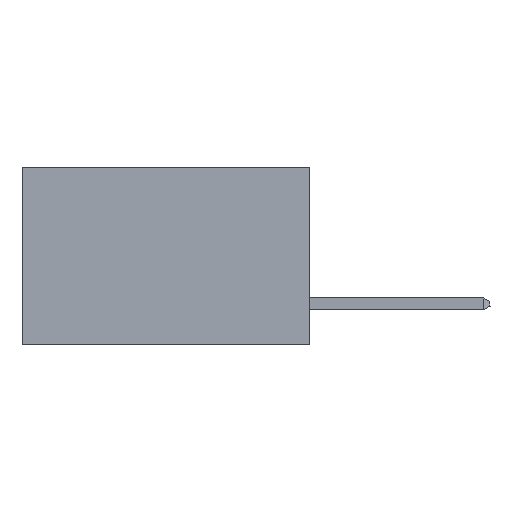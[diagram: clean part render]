
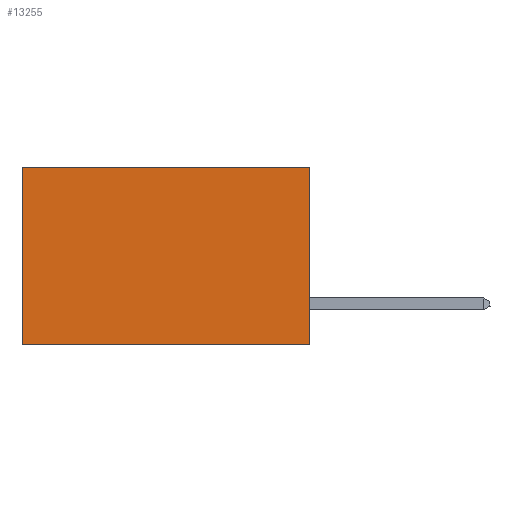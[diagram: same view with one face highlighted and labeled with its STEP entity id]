
A CAD part, left-side view. The second image highlights one B-rep face of the part: STEP entity #13255.
In plain terms, the highlighted planar face has unit normal (-1, 0, 0).
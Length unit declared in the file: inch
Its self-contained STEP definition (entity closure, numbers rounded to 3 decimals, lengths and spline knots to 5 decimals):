
#263 = LINE ( 'NONE', #4884, #8646 ) ;
#336 = VERTEX_POINT ( 'NONE', #20911 ) ;
#1980 = VECTOR ( 'NONE', #3413, 39.37008 ) ;
#2039 = VERTEX_POINT ( 'NONE', #3823 ) ;
#2098 = FACE_OUTER_BOUND ( 'NONE', #17016, .T. ) ;
#3413 = DIRECTION ( 'NONE',  ( 0., 1., 0. ) ) ;
#3480 = CARTESIAN_POINT ( 'NONE',  ( 0.2875, 0., -0.37 ) ) ;
#3809 = DIRECTION ( 'NONE',  ( 0., 0., -1. ) ) ;
#3823 = CARTESIAN_POINT ( 'NONE',  ( 0.2875, 0.6, -0.37 ) ) ;
#3948 = LINE ( 'NONE', #21448, #16694 ) ;
#4884 = CARTESIAN_POINT ( 'NONE',  ( 0.2875, 0., 0. ) ) ;
#4907 = EDGE_CURVE ( 'NONE', #336, #2039, #6445, .T. ) ;
#5338 = CARTESIAN_POINT ( 'NONE',  ( 0.2875, 0., 0. ) ) ;
#5487 = AXIS2_PLACEMENT_3D ( 'NONE', #18658, #13828, #3809 ) ;
#6445 = LINE ( 'NONE', #3480, #1980 ) ;
#6712 = VECTOR ( 'NONE', #20256, 39.37008 ) ;
#7394 = ORIENTED_EDGE ( 'NONE', *, *, #4907, .F. ) ;
#7807 = EDGE_CURVE ( 'NONE', #16595, #2039, #3948, .T. ) ;
#8358 = DIRECTION ( 'NONE',  ( 0., 0., -1. ) ) ;
#8646 = VECTOR ( 'NONE', #13247, 39.37008 ) ;
#8950 = VERTEX_POINT ( 'NONE', #5338 ) ;
#11802 = ORIENTED_EDGE ( 'NONE', *, *, #13146, .F. ) ;
#12154 = PLANE ( 'NONE',  #5487 ) ;
#13146 = EDGE_CURVE ( 'NONE', #8950, #336, #263, .T. ) ;
#13247 = DIRECTION ( 'NONE',  ( 0., 0., -1. ) ) ;
#13255 = ADVANCED_FACE ( 'NONE', ( #2098 ), #12154, .F. ) ;
#13267 = CARTESIAN_POINT ( 'NONE',  ( 0.2875, 0.6, 0. ) ) ;
#13828 = DIRECTION ( 'NONE',  ( 1., 0., 0. ) ) ;
#13845 = CARTESIAN_POINT ( 'NONE',  ( 0.2875, 0., 0. ) ) ;
#14231 = ORIENTED_EDGE ( 'NONE', *, *, #7807, .T. ) ;
#16106 = LINE ( 'NONE', #13845, #6712 ) ;
#16595 = VERTEX_POINT ( 'NONE', #13267 ) ;
#16694 = VECTOR ( 'NONE', #8358, 39.37008 ) ;
#17016 = EDGE_LOOP ( 'NONE', ( #14231, #7394, #11802, #17606 ) ) ;
#17606 = ORIENTED_EDGE ( 'NONE', *, *, #20630, .T. ) ;
#18658 = CARTESIAN_POINT ( 'NONE',  ( 0.2875, 0., 0. ) ) ;
#20256 = DIRECTION ( 'NONE',  ( 0., 1., 0. ) ) ;
#20630 = EDGE_CURVE ( 'NONE', #8950, #16595, #16106, .T. ) ;
#20911 = CARTESIAN_POINT ( 'NONE',  ( 0.2875, 0., -0.37 ) ) ;
#21448 = CARTESIAN_POINT ( 'NONE',  ( 0.2875, 0.6, 0. ) ) ;
